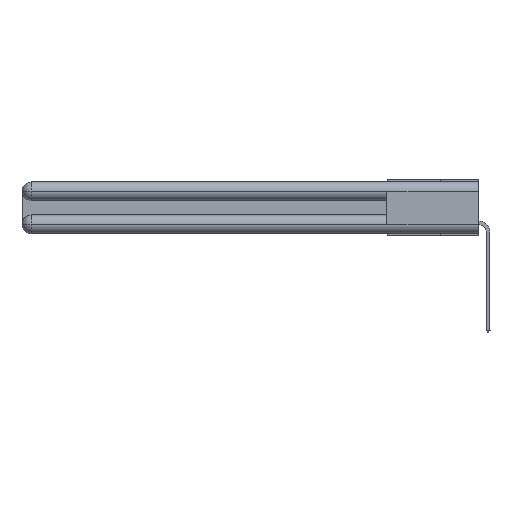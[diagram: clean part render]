
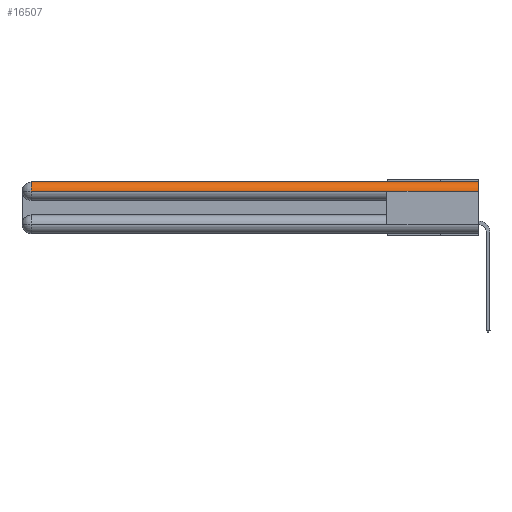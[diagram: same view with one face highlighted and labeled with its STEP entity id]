
A CAD part, left-side view. The second image highlights one B-rep face of the part: STEP entity #16507.
In plain terms, the highlighted cylindrical face has radius 1.562 mm (diameter 3.124 mm), a partial arc.
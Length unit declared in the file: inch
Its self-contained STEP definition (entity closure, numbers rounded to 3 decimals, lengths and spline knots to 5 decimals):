
#322 = CARTESIAN_POINT ( 'NONE',  ( 0.0615, 0., -0.0615 ) ) ;
#393 = EDGE_CURVE ( 'NONE', #23891, #10366, #21928, .T. ) ;
#536 = VERTEX_POINT ( 'NONE', #23160 ) ;
#702 = VECTOR ( 'NONE', #15902, 39.37008 ) ;
#1620 = EDGE_LOOP ( 'NONE', ( #17083, #24044, #10985, #6834, #9994 ) ) ;
#1999 = CYLINDRICAL_SURFACE ( 'NONE', #12746, 0.0615 ) ;
#2306 = CARTESIAN_POINT ( 'NONE',  ( 0., 3., -0.0615 ) ) ;
#2689 = FACE_OUTER_BOUND ( 'NONE', #1620, .T. ) ;
#4021 = DIRECTION ( 'NONE',  ( 1., 0., 0. ) ) ;
#5435 = CARTESIAN_POINT ( 'NONE',  ( 0.0615, 0., 0. ) ) ;
#6434 = AXIS2_PLACEMENT_3D ( 'NONE', #21737, #24745, #26849 ) ;
#6548 = DIRECTION ( 'NONE',  ( 0., 0., 1. ) ) ;
#6828 = CIRCLE ( 'NONE', #19375, 0.0615 ) ;
#6834 = ORIENTED_EDGE ( 'NONE', *, *, #25760, .F. ) ;
#7287 = CIRCLE ( 'NONE', #6434, 0.0615 ) ;
#7329 = CARTESIAN_POINT ( 'NONE',  ( 0.0615, 2.94, 0. ) ) ;
#9994 = ORIENTED_EDGE ( 'NONE', *, *, #15785, .F. ) ;
#10366 = VERTEX_POINT ( 'NONE', #21598 ) ;
#10985 = ORIENTED_EDGE ( 'NONE', *, *, #26242, .T. ) ;
#12362 = LINE ( 'NONE', #22579, #702 ) ;
#12746 = AXIS2_PLACEMENT_3D ( 'NONE', #322, #22005, #6548 ) ;
#12774 = VERTEX_POINT ( 'NONE', #26621 ) ;
#12947 = DIRECTION ( 'NONE',  ( 0., -1., 0. ) ) ;
#12995 = VERTEX_POINT ( 'NONE', #16314 ) ;
#15315 = VECTOR ( 'NONE', #17684, 39.37008 ) ;
#15785 = EDGE_CURVE ( 'NONE', #10366, #536, #6828, .T. ) ;
#15902 = DIRECTION ( 'NONE',  ( 0., 1., 0. ) ) ;
#16314 = CARTESIAN_POINT ( 'NONE',  ( 0., 0.6, -0.0615 ) ) ;
#16507 = ADVANCED_FACE ( 'NONE', ( #2689 ), #1999, .T. ) ;
#17083 = ORIENTED_EDGE ( 'NONE', *, *, #393, .F. ) ;
#17609 = CARTESIAN_POINT ( 'NONE',  ( 0.0615, 0., -0.0615 ) ) ;
#17684 = DIRECTION ( 'NONE',  ( 0., -1., 0. ) ) ;
#19375 = AXIS2_PLACEMENT_3D ( 'NONE', #17609, #12947, #4021 ) ;
#20811 = DIRECTION ( 'NONE',  ( 0., -1., 0. ) ) ;
#21136 = LINE ( 'NONE', #2306, #15315 ) ;
#21598 = CARTESIAN_POINT ( 'NONE',  ( 0.0615, 0., 0. ) ) ;
#21737 = CARTESIAN_POINT ( 'NONE',  ( 0.0615, 2.94, -0.0615 ) ) ;
#21928 = LINE ( 'NONE', #5435, #27726 ) ;
#22005 = DIRECTION ( 'NONE',  ( 0., 1., 0. ) ) ;
#22579 = CARTESIAN_POINT ( 'NONE',  ( 0., 3., -0.0615 ) ) ;
#23160 = CARTESIAN_POINT ( 'NONE',  ( 0., 0., -0.0615 ) ) ;
#23891 = VERTEX_POINT ( 'NONE', #7329 ) ;
#24044 = ORIENTED_EDGE ( 'NONE', *, *, #24313, .T. ) ;
#24313 = EDGE_CURVE ( 'NONE', #23891, #12774, #7287, .T. ) ;
#24745 = DIRECTION ( 'NONE',  ( 0., -1., 0. ) ) ;
#25760 = EDGE_CURVE ( 'NONE', #536, #12995, #12362, .T. ) ;
#26242 = EDGE_CURVE ( 'NONE', #12774, #12995, #21136, .T. ) ;
#26621 = CARTESIAN_POINT ( 'NONE',  ( 0., 2.94, -0.0615 ) ) ;
#26849 = DIRECTION ( 'NONE',  ( 0., 0., 1. ) ) ;
#27726 = VECTOR ( 'NONE', #20811, 39.37008 ) ;
